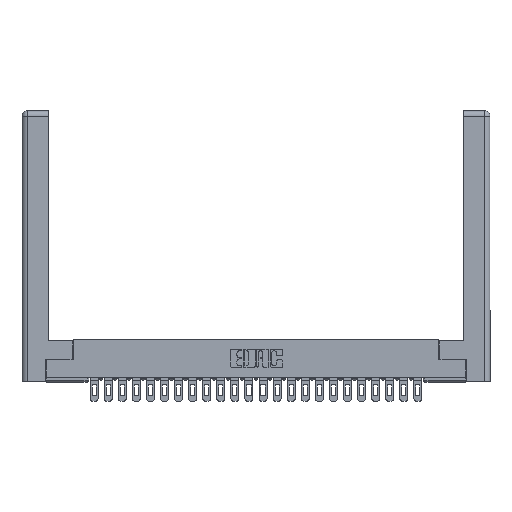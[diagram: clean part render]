
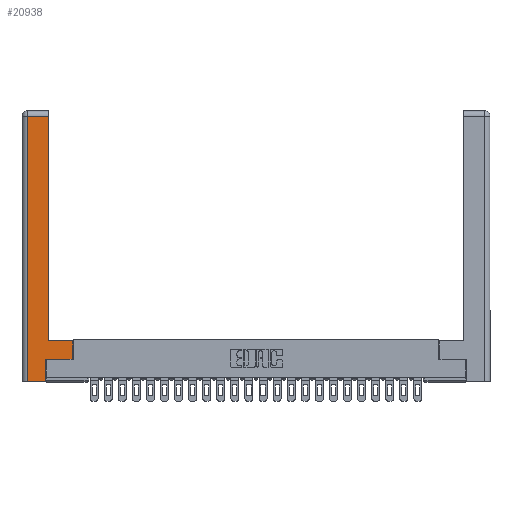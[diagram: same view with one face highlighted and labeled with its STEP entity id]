
A CAD part, top view. The second image highlights one B-rep face of the part: STEP entity #20938.
In plain terms, the highlighted planar face has unit normal (0, 0, 1).
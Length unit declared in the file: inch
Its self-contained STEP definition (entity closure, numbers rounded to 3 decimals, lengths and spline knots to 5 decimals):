
#178 = EDGE_CURVE ( 'NONE', #20630, #12736, #24627, .T. ) ;
#363 = VECTOR ( 'NONE', #4893, 39.37008 ) ;
#564 = DIRECTION ( 'NONE',  ( -1., 0., 0. ) ) ;
#1282 = VERTEX_POINT ( 'NONE', #24791 ) ;
#1308 = CARTESIAN_POINT ( 'NONE',  ( 0.0615, 2.94, 0. ) ) ;
#1614 = VECTOR ( 'NONE', #18975, 39.37008 ) ;
#1927 = CARTESIAN_POINT ( 'NONE',  ( 0., 0., 0. ) ) ;
#2112 = VERTEX_POINT ( 'NONE', #18300 ) ;
#2183 = EDGE_CURVE ( 'NONE', #3179, #2112, #25791, .T. ) ;
#2466 = DIRECTION ( 'NONE',  ( -1., 0., 0. ) ) ;
#3163 = VECTOR ( 'NONE', #564, 39.37008 ) ;
#3179 = VERTEX_POINT ( 'NONE', #19741 ) ;
#3581 = LINE ( 'NONE', #20963, #363 ) ;
#3664 = DIRECTION ( 'NONE',  ( 1., 0., 0. ) ) ;
#4893 = DIRECTION ( 'NONE',  ( 0., -1., 0. ) ) ;
#5595 = ORIENTED_EDGE ( 'NONE', *, *, #21755, .T. ) ;
#5843 = CARTESIAN_POINT ( 'NONE',  ( 0.295, 3., 0. ) ) ;
#5952 = CARTESIAN_POINT ( 'NONE',  ( 0.265, 0., 0. ) ) ;
#6540 = CARTESIAN_POINT ( 'NONE',  ( 0.295, 2.94, 0. ) ) ;
#6944 = LINE ( 'NONE', #5843, #24952 ) ;
#7104 = LINE ( 'NONE', #18374, #17836 ) ;
#7248 = ORIENTED_EDGE ( 'NONE', *, *, #25136, .T. ) ;
#7838 = CARTESIAN_POINT ( 'NONE',  ( 0.0615, 0., 0. ) ) ;
#8424 = DIRECTION ( 'NONE',  ( -1., 0., 0. ) ) ;
#8695 = ORIENTED_EDGE ( 'NONE', *, *, #14066, .T. ) ;
#8976 = ORIENTED_EDGE ( 'NONE', *, *, #25131, .T. ) ;
#9643 = VERTEX_POINT ( 'NONE', #17649 ) ;
#11055 = ORIENTED_EDGE ( 'NONE', *, *, #178, .T. ) ;
#12100 = DIRECTION ( 'NONE',  ( 0., 1., 0. ) ) ;
#12698 = CARTESIAN_POINT ( 'NONE',  ( 0.0615, 2.94, 0. ) ) ;
#12736 = VERTEX_POINT ( 'NONE', #1308 ) ;
#13096 = EDGE_CURVE ( 'NONE', #26240, #3179, #25324, .T. ) ;
#13261 = ORIENTED_EDGE ( 'NONE', *, *, #13096, .T. ) ;
#14061 = CARTESIAN_POINT ( 'NONE',  ( 0.565, 0.245, 0. ) ) ;
#14066 = EDGE_CURVE ( 'NONE', #16804, #26240, #19879, .T. ) ;
#15845 = CARTESIAN_POINT ( 'NONE',  ( 0.265, 0., 0. ) ) ;
#16143 = DIRECTION ( 'NONE',  ( 0., 0., -1. ) ) ;
#16397 = ORIENTED_EDGE ( 'NONE', *, *, #2183, .T. ) ;
#16804 = VERTEX_POINT ( 'NONE', #7838 ) ;
#16906 = VECTOR ( 'NONE', #8424, 39.37008 ) ;
#17649 = CARTESIAN_POINT ( 'NONE',  ( 0.565, 0.45, 0. ) ) ;
#17836 = VECTOR ( 'NONE', #12100, 39.37008 ) ;
#18200 = CARTESIAN_POINT ( 'NONE',  ( 0.295, 0.45, 0. ) ) ;
#18300 = CARTESIAN_POINT ( 'NONE',  ( 0.565, 0.245, 0. ) ) ;
#18374 = CARTESIAN_POINT ( 'NONE',  ( 0.565, 0.45, 0. ) ) ;
#18975 = DIRECTION ( 'NONE',  ( 0., 1., 0. ) ) ;
#19741 = CARTESIAN_POINT ( 'NONE',  ( 0.265, 0.245, 0. ) ) ;
#19879 = LINE ( 'NONE', #5952, #26184 ) ;
#20188 = EDGE_CURVE ( 'NONE', #12736, #16804, #3581, .T. ) ;
#20630 = VERTEX_POINT ( 'NONE', #6540 ) ;
#20763 = VECTOR ( 'NONE', #22518, 39.37008 ) ;
#20938 = ADVANCED_FACE ( 'NONE', ( #24695 ), #22042, .F. ) ;
#20963 = CARTESIAN_POINT ( 'NONE',  ( 0.0615, 0., 0. ) ) ;
#21097 = CARTESIAN_POINT ( 'NONE',  ( 0.265, 0.245, 0. ) ) ;
#21755 = EDGE_CURVE ( 'NONE', #1282, #20630, #6944, .T. ) ;
#21848 = AXIS2_PLACEMENT_3D ( 'NONE', #1927, #16143, #2466 ) ;
#22042 = PLANE ( 'NONE',  #21848 ) ;
#22518 = DIRECTION ( 'NONE',  ( 1., 0., 0. ) ) ;
#22784 = EDGE_LOOP ( 'NONE', ( #5595, #11055, #25244, #8695, #13261, #16397, #7248, #8976 ) ) ;
#23530 = LINE ( 'NONE', #18200, #16906 ) ;
#24627 = LINE ( 'NONE', #12698, #3163 ) ;
#24695 = FACE_OUTER_BOUND ( 'NONE', #22784, .T. ) ;
#24791 = CARTESIAN_POINT ( 'NONE',  ( 0.295, 0.45, 0. ) ) ;
#24952 = VECTOR ( 'NONE', #26062, 39.37008 ) ;
#25131 = EDGE_CURVE ( 'NONE', #9643, #1282, #23530, .T. ) ;
#25136 = EDGE_CURVE ( 'NONE', #2112, #9643, #7104, .T. ) ;
#25244 = ORIENTED_EDGE ( 'NONE', *, *, #20188, .T. ) ;
#25324 = LINE ( 'NONE', #21097, #1614 ) ;
#25791 = LINE ( 'NONE', #14061, #20763 ) ;
#26062 = DIRECTION ( 'NONE',  ( 0., 1., 0. ) ) ;
#26184 = VECTOR ( 'NONE', #3664, 39.37008 ) ;
#26240 = VERTEX_POINT ( 'NONE', #15845 ) ;
